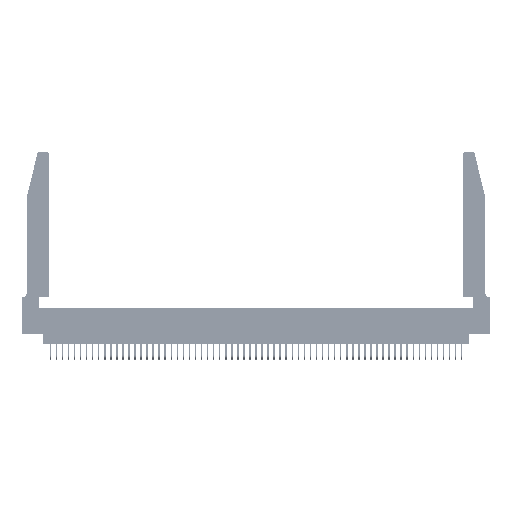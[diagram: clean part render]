
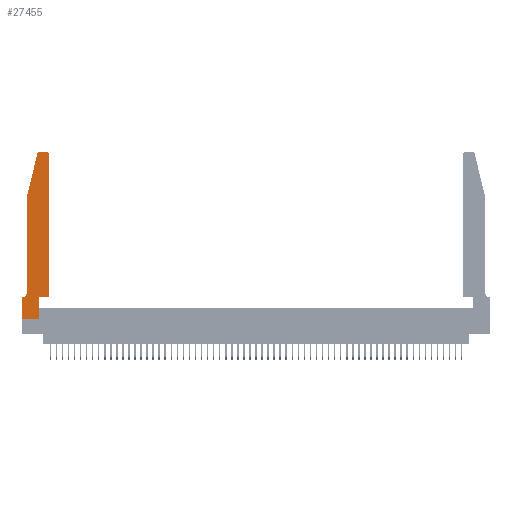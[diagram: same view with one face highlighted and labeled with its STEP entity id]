
A CAD part, top view. The second image highlights one B-rep face of the part: STEP entity #27455.
In plain terms, the highlighted planar face has unit normal (0, 0, 1).
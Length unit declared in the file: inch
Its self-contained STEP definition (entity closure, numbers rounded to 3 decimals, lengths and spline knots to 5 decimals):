
#694 = CARTESIAN_POINT ( 'NONE',  ( 0.4505, 0.35, 0.37 ) ) ;
#901 = ORIENTED_EDGE ( 'NONE', *, *, #43912, .T. ) ;
#4911 = VECTOR ( 'NONE', #17876, 39.37008 ) ;
#4971 = DIRECTION ( 'NONE',  ( -1., 0., 0. ) ) ;
#5397 = VERTEX_POINT ( 'NONE', #32519 ) ;
#5448 = CARTESIAN_POINT ( 'NONE',  ( 0.284, 2.75, 0.37 ) ) ;
#5724 = CARTESIAN_POINT ( 'NONE',  ( 0.25487, 2.72718, 0.37 ) ) ;
#6186 = ORIENTED_EDGE ( 'NONE', *, *, #23857, .T. ) ;
#7187 = CARTESIAN_POINT ( 'NONE',  ( 0.0755, 2., 0.37 ) ) ;
#7486 = EDGE_CURVE ( 'NONE', #46795, #24715, #10950, .T. ) ;
#7560 = LINE ( 'NONE', #20707, #37194 ) ;
#7854 = VERTEX_POINT ( 'NONE', #50193 ) ;
#8024 = DIRECTION ( 'NONE',  ( 1., 0., 0. ) ) ;
#8152 = CARTESIAN_POINT ( 'NONE',  ( 0.4505, 0.35, 0.37 ) ) ;
#8411 = DIRECTION ( 'NONE',  ( 0., 0., 1. ) ) ;
#9179 = EDGE_CURVE ( 'NONE', #53549, #46449, #23791, .T. ) ;
#10950 = CIRCLE ( 'NONE', #13695, 0.03 ) ;
#11613 = DIRECTION ( 'NONE',  ( -0.239, -0.971, 0. ) ) ;
#12159 = ORIENTED_EDGE ( 'NONE', *, *, #21297, .T. ) ;
#12406 = DIRECTION ( 'NONE',  ( 0., 1., 0. ) ) ;
#13695 = AXIS2_PLACEMENT_3D ( 'NONE', #25951, #8411, #30959 ) ;
#13894 = ORIENTED_EDGE ( 'NONE', *, *, #15294, .T. ) ;
#14366 = ORIENTED_EDGE ( 'NONE', *, *, #46043, .T. ) ;
#14946 = CARTESIAN_POINT ( 'NONE',  ( 0.4205, 2.75, 0.37 ) ) ;
#14962 = VERTEX_POINT ( 'NONE', #49033 ) ;
#15294 = EDGE_CURVE ( 'NONE', #24715, #19372, #42763, .T. ) ;
#15702 = CARTESIAN_POINT ( 'NONE',  ( 0.4505, 2.72, 0.37 ) ) ;
#16043 = VERTEX_POINT ( 'NONE', #14946 ) ;
#16283 = CARTESIAN_POINT ( 'NONE',  ( 0.2865, 0.35, 0.37 ) ) ;
#16643 = LINE ( 'NONE', #694, #4911 ) ;
#16812 = CARTESIAN_POINT ( 'NONE',  ( 0., 0.35, 0.37 ) ) ;
#17876 = DIRECTION ( 'NONE',  ( 1., 0., 0. ) ) ;
#19064 = DIRECTION ( 'NONE',  ( 1., 0., 0. ) ) ;
#19194 = VERTEX_POINT ( 'NONE', #51783 ) ;
#19372 = VERTEX_POINT ( 'NONE', #46160 ) ;
#19384 = LINE ( 'NONE', #49640, #48340 ) ;
#20072 = AXIS2_PLACEMENT_3D ( 'NONE', #56362, #34590, #8024 ) ;
#20117 = CARTESIAN_POINT ( 'NONE',  ( 0.0055, 0.42, 0.37 ) ) ;
#20707 = CARTESIAN_POINT ( 'NONE',  ( 0.0755, 0.35, 0.37 ) ) ;
#20825 = DIRECTION ( 'NONE',  ( 0., 0., 1. ) ) ;
#21297 = EDGE_CURVE ( 'NONE', #16043, #46795, #19384, .T. ) ;
#21562 = EDGE_LOOP ( 'NONE', ( #12159, #32316, #13894, #23318, #50343, #27148, #901, #40640, #43290, #14366, #36881, #6186 ) ) ;
#21618 = AXIS2_PLACEMENT_3D ( 'NONE', #20117, #28262, #37088 ) ;
#23318 = ORIENTED_EDGE ( 'NONE', *, *, #45604, .T. ) ;
#23791 = LINE ( 'NONE', #55176, #32753 ) ;
#23857 = EDGE_CURVE ( 'NONE', #43597, #16043, #42569, .T. ) ;
#24715 = VERTEX_POINT ( 'NONE', #5724 ) ;
#25892 = CARTESIAN_POINT ( 'NONE',  ( 0., 0., 0.37 ) ) ;
#25951 = CARTESIAN_POINT ( 'NONE',  ( 0.284, 2.72, 0.37 ) ) ;
#26367 = LINE ( 'NONE', #43793, #27771 ) ;
#27148 = ORIENTED_EDGE ( 'NONE', *, *, #42439, .T. ) ;
#27455 = ADVANCED_FACE ( 'NONE', ( #38085 ), #38171, .T. ) ;
#27771 = VECTOR ( 'NONE', #52442, 39.37008 ) ;
#28262 = DIRECTION ( 'NONE',  ( 0., 0., -1. ) ) ;
#28709 = AXIS2_PLACEMENT_3D ( 'NONE', #16812, #20825, #38939 ) ;
#28823 = DIRECTION ( 'NONE',  ( 0., 1., 0. ) ) ;
#30221 = EDGE_CURVE ( 'NONE', #7854, #53549, #41131, .T. ) ;
#30408 = VECTOR ( 'NONE', #11613, 39.37008 ) ;
#30959 = DIRECTION ( 'NONE',  ( 1., 0., 0. ) ) ;
#31337 = VECTOR ( 'NONE', #12406, 39.37008 ) ;
#32316 = ORIENTED_EDGE ( 'NONE', *, *, #7486, .T. ) ;
#32519 = CARTESIAN_POINT ( 'NONE',  ( 0.4505, 0.35, 0.37 ) ) ;
#32753 = VECTOR ( 'NONE', #28823, 39.37008 ) ;
#32825 = CIRCLE ( 'NONE', #21618, 0.07 ) ;
#33528 = VECTOR ( 'NONE', #19064, 39.37008 ) ;
#33629 = DIRECTION ( 'NONE',  ( -1., 0., 0. ) ) ;
#34590 = DIRECTION ( 'NONE',  ( 0., 0., 1. ) ) ;
#36881 = ORIENTED_EDGE ( 'NONE', *, *, #51944, .T. ) ;
#36904 = VECTOR ( 'NONE', #56693, 39.37008 ) ;
#37088 = DIRECTION ( 'NONE',  ( -1., 0., 0. ) ) ;
#37194 = VECTOR ( 'NONE', #33629, 39.37008 ) ;
#38085 = FACE_OUTER_BOUND ( 'NONE', #21562, .T. ) ;
#38171 = PLANE ( 'NONE',  #28709 ) ;
#38643 = CARTESIAN_POINT ( 'NONE',  ( 0.2865, 0., 0.37 ) ) ;
#38939 = DIRECTION ( 'NONE',  ( 1., 0., 0. ) ) ;
#40640 = ORIENTED_EDGE ( 'NONE', *, *, #30221, .T. ) ;
#40722 = VERTEX_POINT ( 'NONE', #56909 ) ;
#41131 = LINE ( 'NONE', #45428, #33528 ) ;
#41686 = LINE ( 'NONE', #8152, #31337 ) ;
#42439 = EDGE_CURVE ( 'NONE', #40722, #19194, #7560, .T. ) ;
#42569 = CIRCLE ( 'NONE', #20072, 0.03 ) ;
#42763 = LINE ( 'NONE', #7187, #30408 ) ;
#43290 = ORIENTED_EDGE ( 'NONE', *, *, #9179, .T. ) ;
#43582 = EDGE_CURVE ( 'NONE', #14962, #40722, #32825, .T. ) ;
#43597 = VERTEX_POINT ( 'NONE', #15702 ) ;
#43793 = CARTESIAN_POINT ( 'NONE',  ( 0.0755, 2., 0.37 ) ) ;
#43912 = EDGE_CURVE ( 'NONE', #19194, #7854, #45855, .T. ) ;
#45428 = CARTESIAN_POINT ( 'NONE',  ( 0., 0., 0.37 ) ) ;
#45604 = EDGE_CURVE ( 'NONE', #19372, #14962, #26367, .T. ) ;
#45855 = LINE ( 'NONE', #25892, #36904 ) ;
#46043 = EDGE_CURVE ( 'NONE', #46449, #5397, #16643, .T. ) ;
#46160 = CARTESIAN_POINT ( 'NONE',  ( 0.0755, 2., 0.37 ) ) ;
#46449 = VERTEX_POINT ( 'NONE', #16283 ) ;
#46795 = VERTEX_POINT ( 'NONE', #5448 ) ;
#48340 = VECTOR ( 'NONE', #4971, 39.37008 ) ;
#49033 = CARTESIAN_POINT ( 'NONE',  ( 0.0755, 0.42, 0.37 ) ) ;
#49640 = CARTESIAN_POINT ( 'NONE',  ( 0.2605, 2.75, 0.37 ) ) ;
#50193 = CARTESIAN_POINT ( 'NONE',  ( 0., 0., 0.37 ) ) ;
#50343 = ORIENTED_EDGE ( 'NONE', *, *, #43582, .T. ) ;
#51783 = CARTESIAN_POINT ( 'NONE',  ( 0., 0.35, 0.37 ) ) ;
#51944 = EDGE_CURVE ( 'NONE', #5397, #43597, #41686, .T. ) ;
#52442 = DIRECTION ( 'NONE',  ( 0., -1., 0. ) ) ;
#53549 = VERTEX_POINT ( 'NONE', #38643 ) ;
#55176 = CARTESIAN_POINT ( 'NONE',  ( 0.2865, 0.35, 0.37 ) ) ;
#56362 = CARTESIAN_POINT ( 'NONE',  ( 0.4205, 2.72, 0.37 ) ) ;
#56693 = DIRECTION ( 'NONE',  ( 0., -1., 0. ) ) ;
#56909 = CARTESIAN_POINT ( 'NONE',  ( 0.0055, 0.35, 0.37 ) ) ;
